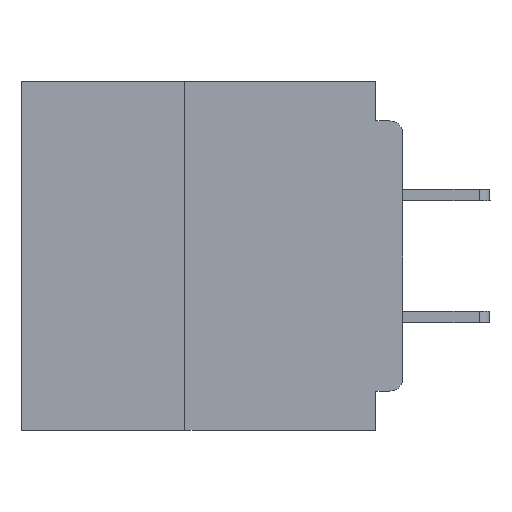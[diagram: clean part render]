
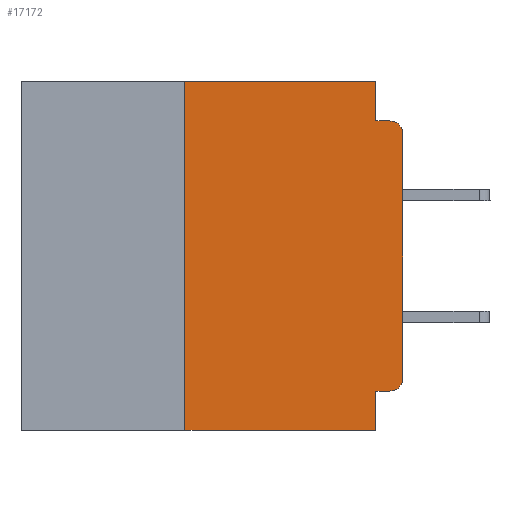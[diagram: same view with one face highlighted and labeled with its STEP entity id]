
A CAD part, left-side view. The second image highlights one B-rep face of the part: STEP entity #17172.
In plain terms, the highlighted planar face has unit normal (-1, 0, 0).
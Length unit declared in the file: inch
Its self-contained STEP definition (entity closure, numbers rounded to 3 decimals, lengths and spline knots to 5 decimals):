
#1848 = ORIENTED_EDGE ( 'NONE', *, *, #35897, .F. ) ;
#2276 = DIRECTION ( 'NONE',  ( -1., 0., 0. ) ) ;
#4108 = AXIS2_PLACEMENT_3D ( 'NONE', #5918, #46273, #16164 ) ;
#5479 = DIRECTION ( 'NONE',  ( 0., -1., 0. ) ) ;
#5918 = CARTESIAN_POINT ( 'NONE',  ( 0., 0.437, 0. ) ) ;
#6715 = CARTESIAN_POINT ( 'NONE',  ( 0., 0.015, -0.34 ) ) ;
#7159 = DIRECTION ( 'NONE',  ( 0., 0., -1. ) ) ;
#7442 = ORIENTED_EDGE ( 'NONE', *, *, #32328, .T. ) ;
#8791 = EDGE_CURVE ( 'NONE', #19141, #62472, #56062, .T. ) ;
#10442 = CARTESIAN_POINT ( 'NONE',  ( 0., 0.437, -0.4 ) ) ;
#10650 = ORIENTED_EDGE ( 'NONE', *, *, #13055, .F. ) ;
#10742 = CARTESIAN_POINT ( 'NONE',  ( 0., 0.031, -0.4 ) ) ;
#10925 = ORIENTED_EDGE ( 'NONE', *, *, #8791, .F. ) ;
#11868 = DIRECTION ( 'NONE',  ( 0., 0., -1. ) ) ;
#13055 = EDGE_CURVE ( 'NONE', #46432, #46823, #31201, .T. ) ;
#13182 = CARTESIAN_POINT ( 'NONE',  ( 0., 0., -0.06 ) ) ;
#14155 = CARTESIAN_POINT ( 'NONE',  ( 0., 0.031, 0. ) ) ;
#14998 = CARTESIAN_POINT ( 'NONE',  ( 0., 0., -0.355 ) ) ;
#15107 = CARTESIAN_POINT ( 'NONE',  ( 0., 0.25, -0.4 ) ) ;
#15677 = CIRCLE ( 'NONE', #28586, 0.015 ) ;
#16164 = DIRECTION ( 'NONE',  ( 0., 0., -1. ) ) ;
#17172 = ADVANCED_FACE ( 'NONE', ( #28504 ), #60924, .F. ) ;
#19141 = VERTEX_POINT ( 'NONE', #62225 ) ;
#21756 = VERTEX_POINT ( 'NONE', #41432 ) ;
#22381 = DIRECTION ( 'NONE',  ( 0., -1., 0. ) ) ;
#22732 = CARTESIAN_POINT ( 'NONE',  ( 0., 0.437, 0. ) ) ;
#23627 = ORIENTED_EDGE ( 'NONE', *, *, #44835, .T. ) ;
#23995 = CARTESIAN_POINT ( 'NONE',  ( 0., 0.015, -0.355 ) ) ;
#24625 = LINE ( 'NONE', #47418, #51344 ) ;
#24895 = DIRECTION ( 'NONE',  ( 0., 1., 0. ) ) ;
#25214 = VECTOR ( 'NONE', #51735, 39.37008 ) ;
#25940 = VECTOR ( 'NONE', #24895, 39.37008 ) ;
#27741 = VERTEX_POINT ( 'NONE', #65043 ) ;
#27980 = VERTEX_POINT ( 'NONE', #36246 ) ;
#28504 = FACE_OUTER_BOUND ( 'NONE', #34700, .T. ) ;
#28586 = AXIS2_PLACEMENT_3D ( 'NONE', #6715, #42020, #11868 ) ;
#29463 = ORIENTED_EDGE ( 'NONE', *, *, #62897, .F. ) ;
#31001 = VECTOR ( 'NONE', #7159, 39.37008 ) ;
#31201 = LINE ( 'NONE', #22732, #43000 ) ;
#32328 = EDGE_CURVE ( 'NONE', #39410, #27741, #59135, .T. ) ;
#32587 = CARTESIAN_POINT ( 'NONE',  ( 0., 0.015, -0.06 ) ) ;
#33442 = DIRECTION ( 'NONE',  ( 0., 0., 1. ) ) ;
#34700 = EDGE_LOOP ( 'NONE', ( #44182, #7442, #29463, #1848, #10650, #38056, #62872, #10925, #64231, #23627 ) ) ;
#35897 = EDGE_CURVE ( 'NONE', #46823, #27980, #45623, .T. ) ;
#35996 = EDGE_CURVE ( 'NONE', #53835, #19141, #54205, .T. ) ;
#36246 = CARTESIAN_POINT ( 'NONE',  ( 0., 0.031, -0.045 ) ) ;
#37666 = DIRECTION ( 'NONE',  ( 0., 0., -1. ) ) ;
#38056 = ORIENTED_EDGE ( 'NONE', *, *, #57849, .F. ) ;
#39410 = VERTEX_POINT ( 'NONE', #13182 ) ;
#41432 = CARTESIAN_POINT ( 'NONE',  ( 0., 0., -0.34 ) ) ;
#42020 = DIRECTION ( 'NONE',  ( -1., 0., 0. ) ) ;
#42452 = CARTESIAN_POINT ( 'NONE',  ( 0., 0.031, -0.4 ) ) ;
#43000 = VECTOR ( 'NONE', #52786, 39.37008 ) ;
#43338 = CARTESIAN_POINT ( 'NONE',  ( 0., 0.25, 0. ) ) ;
#44182 = ORIENTED_EDGE ( 'NONE', *, *, #56703, .T. ) ;
#44835 = EDGE_CURVE ( 'NONE', #53835, #21756, #15677, .T. ) ;
#45623 = LINE ( 'NONE', #14155, #58935 ) ;
#46155 = CARTESIAN_POINT ( 'NONE',  ( 0., 0.031, 0. ) ) ;
#46273 = DIRECTION ( 'NONE',  ( 1., 0., 0. ) ) ;
#46432 = VERTEX_POINT ( 'NONE', #43338 ) ;
#46681 = CARTESIAN_POINT ( 'NONE',  ( 0., 0.25, -0.4 ) ) ;
#46823 = VERTEX_POINT ( 'NONE', #46155 ) ;
#47418 = CARTESIAN_POINT ( 'NONE',  ( 0., 0., -0.045 ) ) ;
#49304 = DIRECTION ( 'NONE',  ( 0., 0., -1. ) ) ;
#49316 = VECTOR ( 'NONE', #33442, 39.37008 ) ;
#51344 = VECTOR ( 'NONE', #22381, 39.37008 ) ;
#51735 = DIRECTION ( 'NONE',  ( 0., 0., 1. ) ) ;
#51933 = LINE ( 'NONE', #46681, #25214 ) ;
#52703 = VERTEX_POINT ( 'NONE', #15107 ) ;
#52786 = DIRECTION ( 'NONE',  ( 0., -1., 0. ) ) ;
#53835 = VERTEX_POINT ( 'NONE', #23995 ) ;
#54205 = LINE ( 'NONE', #14998, #25940 ) ;
#55176 = LINE ( 'NONE', #10442, #56750 ) ;
#56062 = LINE ( 'NONE', #42452, #31001 ) ;
#56703 = EDGE_CURVE ( 'NONE', #21756, #39410, #59474, .T. ) ;
#56750 = VECTOR ( 'NONE', #5479, 39.37008 ) ;
#57849 = EDGE_CURVE ( 'NONE', #52703, #46432, #51933, .T. ) ;
#58935 = VECTOR ( 'NONE', #49304, 39.37008 ) ;
#59135 = CIRCLE ( 'NONE', #62131, 0.015 ) ;
#59474 = LINE ( 'NONE', #63449, #49316 ) ;
#60924 = PLANE ( 'NONE',  #4108 ) ;
#62131 = AXIS2_PLACEMENT_3D ( 'NONE', #32587, #2276, #37666 ) ;
#62225 = CARTESIAN_POINT ( 'NONE',  ( 0., 0.031, -0.355 ) ) ;
#62472 = VERTEX_POINT ( 'NONE', #10742 ) ;
#62872 = ORIENTED_EDGE ( 'NONE', *, *, #65173, .T. ) ;
#62897 = EDGE_CURVE ( 'NONE', #27980, #27741, #24625, .T. ) ;
#63449 = CARTESIAN_POINT ( 'NONE',  ( 0., 0., 0. ) ) ;
#64231 = ORIENTED_EDGE ( 'NONE', *, *, #35996, .F. ) ;
#65043 = CARTESIAN_POINT ( 'NONE',  ( 0., 0.015, -0.045 ) ) ;
#65173 = EDGE_CURVE ( 'NONE', #52703, #62472, #55176, .T. ) ;
